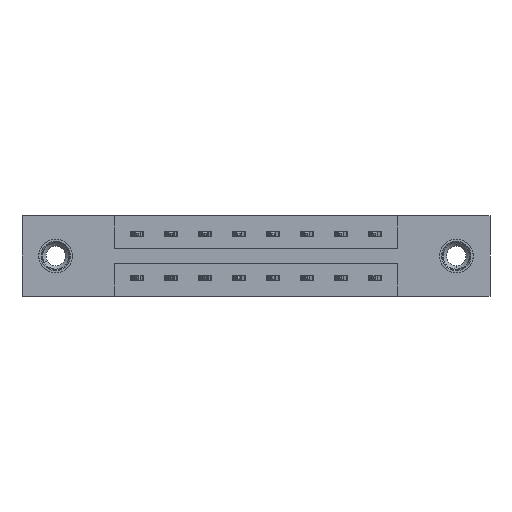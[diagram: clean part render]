
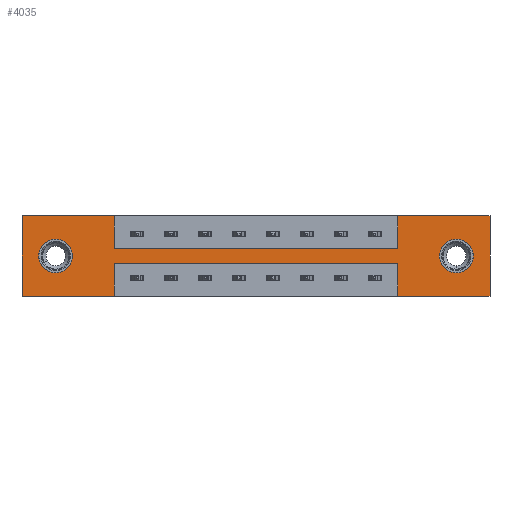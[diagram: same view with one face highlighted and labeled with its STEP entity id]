
A CAD part, front view. The second image highlights one B-rep face of the part: STEP entity #4035.
In plain terms, the highlighted planar face has unit normal (0, -1, 0).
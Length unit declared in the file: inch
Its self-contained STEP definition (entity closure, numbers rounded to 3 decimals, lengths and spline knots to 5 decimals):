
#98 = CARTESIAN_POINT ( 'NONE',  ( 0.425, 0., -0.22 ) ) ;
#147 = PLANE ( 'NONE',  #10394 ) ;
#191 = ORIENTED_EDGE ( 'NONE', *, *, #4256, .T. ) ;
#330 = FACE_BOUND ( 'NONE', #6625, .T. ) ;
#361 = CARTESIAN_POINT ( 'NONE',  ( 0.155, 0., -0.107 ) ) ;
#536 = ORIENTED_EDGE ( 'NONE', *, *, #1426, .F. ) ;
#545 = VECTOR ( 'NONE', #7456, 39.37008 ) ;
#616 = EDGE_CURVE ( 'NONE', #11796, #2792, #9761, .T. ) ;
#646 = LINE ( 'NONE', #7626, #5514 ) ;
#665 = FACE_BOUND ( 'NONE', #2684, .T. ) ;
#823 = AXIS2_PLACEMENT_3D ( 'NONE', #3069, #4104, #7678 ) ;
#828 = ORIENTED_EDGE ( 'NONE', *, *, #1329, .F. ) ;
#885 = CARTESIAN_POINT ( 'NONE',  ( 0.425, 0., -0.37 ) ) ;
#928 = CARTESIAN_POINT ( 'NONE',  ( 0.425, 0., 0. ) ) ;
#972 = VERTEX_POINT ( 'NONE', #10159 ) ;
#980 = VECTOR ( 'NONE', #10672, 39.37008 ) ;
#1127 = ORIENTED_EDGE ( 'NONE', *, *, #2361, .F. ) ;
#1226 = CARTESIAN_POINT ( 'NONE',  ( 0.155, 0., -0.263 ) ) ;
#1251 = EDGE_CURVE ( 'NONE', #2069, #10588, #8158, .T. ) ;
#1290 = EDGE_CURVE ( 'NONE', #8253, #7767, #7355, .T. ) ;
#1293 = LINE ( 'NONE', #10267, #980 ) ;
#1329 = EDGE_CURVE ( 'NONE', #7767, #6264, #1617, .T. ) ;
#1367 = EDGE_CURVE ( 'NONE', #11521, #2069, #1293, .T. ) ;
#1403 = EDGE_CURVE ( 'NONE', #2108, #6851, #3048, .T. ) ;
#1407 = EDGE_CURVE ( 'NONE', #5823, #11521, #7744, .T. ) ;
#1426 = EDGE_CURVE ( 'NONE', #11397, #5823, #7213, .T. ) ;
#1431 = EDGE_CURVE ( 'NONE', #6264, #11397, #4950, .T. ) ;
#1445 = EDGE_CURVE ( 'NONE', #8851, #6107, #1765, .T. ) ;
#1446 = EDGE_CURVE ( 'NONE', #972, #8851, #11140, .T. ) ;
#1448 = LINE ( 'NONE', #10664, #8654 ) ;
#1464 = EDGE_CURVE ( 'NONE', #2406, #972, #1448, .T. ) ;
#1592 = EDGE_CURVE ( 'NONE', #6851, #2108, #3927, .T. ) ;
#1617 = LINE ( 'NONE', #7003, #11016 ) ;
#1765 = LINE ( 'NONE', #8139, #6648 ) ;
#1993 = CARTESIAN_POINT ( 'NONE',  ( 2.154, 0., 0. ) ) ;
#2047 = CARTESIAN_POINT ( 'NONE',  ( 2.154, 0., -0.37 ) ) ;
#2069 = VERTEX_POINT ( 'NONE', #5236 ) ;
#2093 = VECTOR ( 'NONE', #9061, 39.37008 ) ;
#2108 = VERTEX_POINT ( 'NONE', #3756 ) ;
#2185 = DIRECTION ( 'NONE',  ( 0., 0., -1. ) ) ;
#2280 = EDGE_CURVE ( 'NONE', #10588, #2406, #9850, .T. ) ;
#2361 = EDGE_CURVE ( 'NONE', #6107, #8253, #646, .T. ) ;
#2406 = VERTEX_POINT ( 'NONE', #928 ) ;
#2534 = VECTOR ( 'NONE', #3699, 39.37008 ) ;
#2575 = ORIENTED_EDGE ( 'NONE', *, *, #1403, .T. ) ;
#2582 = VECTOR ( 'NONE', #10262, 39.37008 ) ;
#2684 = EDGE_LOOP ( 'NONE', ( #2575, #7613 ) ) ;
#2693 = CARTESIAN_POINT ( 'NONE',  ( 1.729, 0., 0. ) ) ;
#2711 = CARTESIAN_POINT ( 'NONE',  ( 0., 0., 0. ) ) ;
#2766 = DIRECTION ( 'NONE',  ( 0., 1., 0. ) ) ;
#2792 = VERTEX_POINT ( 'NONE', #361 ) ;
#2889 = ORIENTED_EDGE ( 'NONE', *, *, #616, .T. ) ;
#3048 = CIRCLE ( 'NONE', #3754, 0.078 ) ;
#3069 = CARTESIAN_POINT ( 'NONE',  ( 1.999, 0., -0.185 ) ) ;
#3291 = EDGE_LOOP ( 'NONE', ( #10147, #536, #10402, #828, #3510, #1127, #8659, #8934, #6949, #9055, #11249, #4497 ) ) ;
#3510 = ORIENTED_EDGE ( 'NONE', *, *, #1290, .F. ) ;
#3699 = DIRECTION ( 'NONE',  ( 1., 0., 0. ) ) ;
#3703 = CARTESIAN_POINT ( 'NONE',  ( 1.729, 0., -0.15 ) ) ;
#3754 = AXIS2_PLACEMENT_3D ( 'NONE', #3787, #2766, #10794 ) ;
#3756 = CARTESIAN_POINT ( 'NONE',  ( 1.999, 0., -0.107 ) ) ;
#3787 = CARTESIAN_POINT ( 'NONE',  ( 1.999, 0., -0.185 ) ) ;
#3927 = CIRCLE ( 'NONE', #823, 0.078 ) ;
#3972 = CARTESIAN_POINT ( 'NONE',  ( 0.425, 0., -0.37 ) ) ;
#4035 = ADVANCED_FACE ( 'NONE', ( #665, #330, #10251 ), #147, .T. ) ;
#4104 = DIRECTION ( 'NONE',  ( 0., 1., 0. ) ) ;
#4256 = EDGE_CURVE ( 'NONE', #2792, #11796, #11359, .T. ) ;
#4496 = DIRECTION ( 'NONE',  ( 0., 1., 0. ) ) ;
#4497 = ORIENTED_EDGE ( 'NONE', *, *, #1367, .F. ) ;
#4782 = CARTESIAN_POINT ( 'NONE',  ( 1.729, 0., -0.22 ) ) ;
#4854 = CARTESIAN_POINT ( 'NONE',  ( 1.729, 0., -0.37 ) ) ;
#4912 = CARTESIAN_POINT ( 'NONE',  ( 0.425, 0., -0.22 ) ) ;
#4950 = LINE ( 'NONE', #9965, #6943 ) ;
#5236 = CARTESIAN_POINT ( 'NONE',  ( 0., 0., -0.37 ) ) ;
#5514 = VECTOR ( 'NONE', #8492, 39.37008 ) ;
#5823 = VERTEX_POINT ( 'NONE', #98 ) ;
#6107 = VERTEX_POINT ( 'NONE', #2693 ) ;
#6264 = VERTEX_POINT ( 'NONE', #4854 ) ;
#6625 = EDGE_LOOP ( 'NONE', ( #191, #2889 ) ) ;
#6648 = VECTOR ( 'NONE', #8293, 39.37008 ) ;
#6688 = CARTESIAN_POINT ( 'NONE',  ( 1.999, 0., -0.263 ) ) ;
#6851 = VERTEX_POINT ( 'NONE', #6688 ) ;
#6943 = VECTOR ( 'NONE', #9220, 39.37008 ) ;
#6949 = ORIENTED_EDGE ( 'NONE', *, *, #1464, .F. ) ;
#7003 = CARTESIAN_POINT ( 'NONE',  ( 0., 0., -0.37 ) ) ;
#7213 = LINE ( 'NONE', #4912, #11386 ) ;
#7355 = LINE ( 'NONE', #1993, #2582 ) ;
#7456 = DIRECTION ( 'NONE',  ( 0., 0., 1. ) ) ;
#7613 = ORIENTED_EDGE ( 'NONE', *, *, #1592, .T. ) ;
#7626 = CARTESIAN_POINT ( 'NONE',  ( 0., 0., 0. ) ) ;
#7678 = DIRECTION ( 'NONE',  ( 0., 0., -1. ) ) ;
#7744 = LINE ( 'NONE', #885, #9752 ) ;
#7767 = VERTEX_POINT ( 'NONE', #2047 ) ;
#7820 = CARTESIAN_POINT ( 'NONE',  ( 0., 0., -0.37 ) ) ;
#7900 = AXIS2_PLACEMENT_3D ( 'NONE', #9903, #4496, #10721 ) ;
#8139 = CARTESIAN_POINT ( 'NONE',  ( 1.729, 0., 0. ) ) ;
#8158 = LINE ( 'NONE', #8419, #545 ) ;
#8253 = VERTEX_POINT ( 'NONE', #10922 ) ;
#8293 = DIRECTION ( 'NONE',  ( 0., 0., 1. ) ) ;
#8419 = CARTESIAN_POINT ( 'NONE',  ( 0., 0., 0. ) ) ;
#8492 = DIRECTION ( 'NONE',  ( 1., 0., 0. ) ) ;
#8654 = VECTOR ( 'NONE', #9128, 39.37008 ) ;
#8659 = ORIENTED_EDGE ( 'NONE', *, *, #1445, .F. ) ;
#8851 = VERTEX_POINT ( 'NONE', #3703 ) ;
#8934 = ORIENTED_EDGE ( 'NONE', *, *, #1446, .F. ) ;
#9055 = ORIENTED_EDGE ( 'NONE', *, *, #2280, .F. ) ;
#9061 = DIRECTION ( 'NONE',  ( 1., 0., 0. ) ) ;
#9128 = DIRECTION ( 'NONE',  ( 0., 0., -1. ) ) ;
#9220 = DIRECTION ( 'NONE',  ( 0., 0., 1. ) ) ;
#9437 = DIRECTION ( 'NONE',  ( 0., 0., -1. ) ) ;
#9479 = DIRECTION ( 'NONE',  ( -1., 0., 0. ) ) ;
#9752 = VECTOR ( 'NONE', #9437, 39.37008 ) ;
#9761 = CIRCLE ( 'NONE', #9888, 0.078 ) ;
#9850 = LINE ( 'NONE', #2711, #2534 ) ;
#9888 = AXIS2_PLACEMENT_3D ( 'NONE', #10371, #11312, #11364 ) ;
#9903 = CARTESIAN_POINT ( 'NONE',  ( 0.155, 0., -0.185 ) ) ;
#9956 = CARTESIAN_POINT ( 'NONE',  ( 0.425, 0., -0.15 ) ) ;
#9965 = CARTESIAN_POINT ( 'NONE',  ( 1.729, 0., -0.37 ) ) ;
#10147 = ORIENTED_EDGE ( 'NONE', *, *, #1407, .F. ) ;
#10159 = CARTESIAN_POINT ( 'NONE',  ( 0.425, 0., -0.15 ) ) ;
#10251 = FACE_OUTER_BOUND ( 'NONE', #3291, .T. ) ;
#10262 = DIRECTION ( 'NONE',  ( 0., 0., -1. ) ) ;
#10267 = CARTESIAN_POINT ( 'NONE',  ( 0., 0., -0.37 ) ) ;
#10371 = CARTESIAN_POINT ( 'NONE',  ( 0.155, 0., -0.185 ) ) ;
#10384 = DIRECTION ( 'NONE',  ( 0., -1., 0. ) ) ;
#10394 = AXIS2_PLACEMENT_3D ( 'NONE', #7820, #10384, #2185 ) ;
#10402 = ORIENTED_EDGE ( 'NONE', *, *, #1431, .F. ) ;
#10588 = VERTEX_POINT ( 'NONE', #11111 ) ;
#10664 = CARTESIAN_POINT ( 'NONE',  ( 0.425, 0., 0. ) ) ;
#10672 = DIRECTION ( 'NONE',  ( -1., 0., 0. ) ) ;
#10721 = DIRECTION ( 'NONE',  ( 0., 0., 1. ) ) ;
#10794 = DIRECTION ( 'NONE',  ( 0., 0., -1. ) ) ;
#10922 = CARTESIAN_POINT ( 'NONE',  ( 2.154, 0., 0. ) ) ;
#11016 = VECTOR ( 'NONE', #11411, 39.37008 ) ;
#11111 = CARTESIAN_POINT ( 'NONE',  ( 0., 0., 0. ) ) ;
#11140 = LINE ( 'NONE', #9956, #2093 ) ;
#11249 = ORIENTED_EDGE ( 'NONE', *, *, #1251, .F. ) ;
#11312 = DIRECTION ( 'NONE',  ( 0., 1., 0. ) ) ;
#11359 = CIRCLE ( 'NONE', #7900, 0.078 ) ;
#11364 = DIRECTION ( 'NONE',  ( 0., 0., 1. ) ) ;
#11386 = VECTOR ( 'NONE', #9479, 39.37008 ) ;
#11397 = VERTEX_POINT ( 'NONE', #4782 ) ;
#11411 = DIRECTION ( 'NONE',  ( -1., 0., 0. ) ) ;
#11521 = VERTEX_POINT ( 'NONE', #3972 ) ;
#11796 = VERTEX_POINT ( 'NONE', #1226 ) ;
